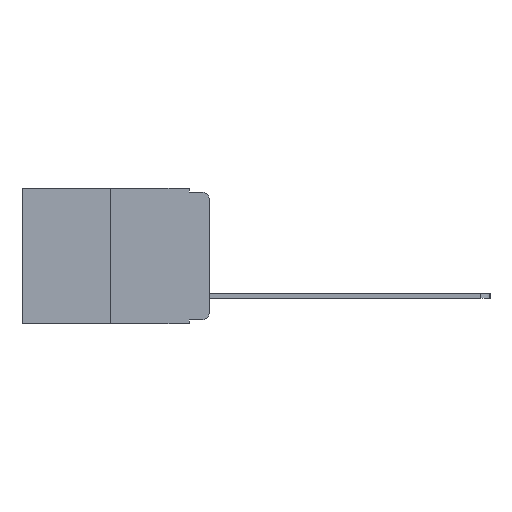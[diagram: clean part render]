
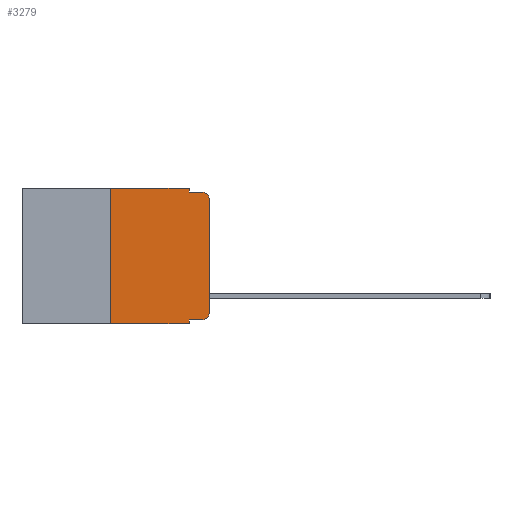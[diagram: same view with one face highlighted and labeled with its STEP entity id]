
A CAD part, left-side view. The second image highlights one B-rep face of the part: STEP entity #3279.
In plain terms, the highlighted planar face has unit normal (-1, 0, 0).
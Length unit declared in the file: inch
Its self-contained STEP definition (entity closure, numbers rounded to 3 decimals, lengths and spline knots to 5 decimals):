
#156 = CARTESIAN_POINT ( 'NONE',  ( 0., 0.02, -0.01 ) ) ;
#535 = ORIENTED_EDGE ( 'NONE', *, *, #969, .T. ) ;
#563 = CARTESIAN_POINT ( 'NONE',  ( 0., 0., -0.03 ) ) ;
#684 = VECTOR ( 'NONE', #9339, 39.37008 ) ;
#969 = EDGE_CURVE ( 'NONE', #7071, #10668, #7395, .T. ) ;
#1156 = VECTOR ( 'NONE', #9310, 39.37008 ) ;
#1168 = CARTESIAN_POINT ( 'NONE',  ( 0., 0.25, 0. ) ) ;
#1169 = VERTEX_POINT ( 'NONE', #3076 ) ;
#1619 = VERTEX_POINT ( 'NONE', #1168 ) ;
#1638 = FACE_OUTER_BOUND ( 'NONE', #4559, .T. ) ;
#1815 = CIRCLE ( 'NONE', #15956, 0.02 ) ;
#1949 = CARTESIAN_POINT ( 'NONE',  ( 0., 0.051, 0. ) ) ;
#2222 = ORIENTED_EDGE ( 'NONE', *, *, #12301, .F. ) ;
#2298 = LINE ( 'NONE', #12365, #6300 ) ;
#2747 = CARTESIAN_POINT ( 'NONE',  ( 0., 0., -0.313 ) ) ;
#2763 = DIRECTION ( 'NONE',  ( -1., 0., 0. ) ) ;
#2856 = LINE ( 'NONE', #8801, #13607 ) ;
#3076 = CARTESIAN_POINT ( 'NONE',  ( 0., 0.051, -0.333 ) ) ;
#3279 = ADVANCED_FACE ( 'NONE', ( #1638 ), #4726, .F. ) ;
#3405 = DIRECTION ( 'NONE',  ( 0., -1., 0. ) ) ;
#4073 = CARTESIAN_POINT ( 'NONE',  ( 0., 0.051, 0. ) ) ;
#4359 = EDGE_CURVE ( 'NONE', #1619, #12230, #13391, .T. ) ;
#4559 = EDGE_LOOP ( 'NONE', ( #16207, #16628, #2222, #13910, #7570, #8015, #535, #16010, #16838, #10166 ) ) ;
#4726 = PLANE ( 'NONE',  #13840 ) ;
#4734 = EDGE_CURVE ( 'NONE', #7071, #1619, #2856, .T. ) ;
#4788 = DIRECTION ( 'NONE',  ( 1., 0., 0. ) ) ;
#5229 = EDGE_CURVE ( 'NONE', #13430, #14707, #1815, .T. ) ;
#5599 = EDGE_CURVE ( 'NONE', #1169, #13430, #2298, .T. ) ;
#6300 = VECTOR ( 'NONE', #13684, 39.37008 ) ;
#6925 = EDGE_CURVE ( 'NONE', #1169, #10668, #13005, .T. ) ;
#7071 = VERTEX_POINT ( 'NONE', #15004 ) ;
#7157 = DIRECTION ( 'NONE',  ( 0., 0., -1. ) ) ;
#7208 = CARTESIAN_POINT ( 'NONE',  ( 0., 0.051, -0.01 ) ) ;
#7281 = LINE ( 'NONE', #12163, #10475 ) ;
#7308 = AXIS2_PLACEMENT_3D ( 'NONE', #16505, #8493, #7157 ) ;
#7395 = LINE ( 'NONE', #14921, #11018 ) ;
#7570 = ORIENTED_EDGE ( 'NONE', *, *, #4359, .F. ) ;
#7743 = CARTESIAN_POINT ( 'NONE',  ( 0., 0.02, -0.333 ) ) ;
#8015 = ORIENTED_EDGE ( 'NONE', *, *, #4734, .F. ) ;
#8082 = EDGE_CURVE ( 'NONE', #17076, #13344, #10045, .T. ) ;
#8493 = DIRECTION ( 'NONE',  ( -1., 0., 0. ) ) ;
#8608 = LINE ( 'NONE', #1949, #684 ) ;
#8801 = CARTESIAN_POINT ( 'NONE',  ( 0., 0.25, 0. ) ) ;
#9310 = DIRECTION ( 'NONE',  ( 0., 0., -1. ) ) ;
#9339 = DIRECTION ( 'NONE',  ( 0., 0., -1. ) ) ;
#10045 = CIRCLE ( 'NONE', #7308, 0.02 ) ;
#10166 = ORIENTED_EDGE ( 'NONE', *, *, #5229, .T. ) ;
#10178 = VERTEX_POINT ( 'NONE', #7208 ) ;
#10475 = VECTOR ( 'NONE', #13488, 39.37008 ) ;
#10668 = VERTEX_POINT ( 'NONE', #10711 ) ;
#10711 = CARTESIAN_POINT ( 'NONE',  ( 0., 0.051, -0.343 ) ) ;
#11018 = VECTOR ( 'NONE', #14616, 39.37008 ) ;
#11313 = CARTESIAN_POINT ( 'NONE',  ( 0., 0.02, -0.313 ) ) ;
#11963 = EDGE_CURVE ( 'NONE', #12230, #10178, #8608, .T. ) ;
#12059 = EDGE_CURVE ( 'NONE', #14707, #17076, #7281, .T. ) ;
#12163 = CARTESIAN_POINT ( 'NONE',  ( 0., 0., 0. ) ) ;
#12230 = VERTEX_POINT ( 'NONE', #4073 ) ;
#12301 = EDGE_CURVE ( 'NONE', #10178, #13344, #17746, .T. ) ;
#12365 = CARTESIAN_POINT ( 'NONE',  ( 0., 0.051, -0.333 ) ) ;
#12659 = DIRECTION ( 'NONE',  ( 0., 0., -1. ) ) ;
#12980 = VECTOR ( 'NONE', #3405, 39.37008 ) ;
#13005 = LINE ( 'NONE', #15967, #1156 ) ;
#13073 = CARTESIAN_POINT ( 'NONE',  ( 0., 0.473, 0. ) ) ;
#13344 = VERTEX_POINT ( 'NONE', #156 ) ;
#13391 = LINE ( 'NONE', #17128, #12980 ) ;
#13430 = VERTEX_POINT ( 'NONE', #7743 ) ;
#13488 = DIRECTION ( 'NONE',  ( 0., 0., 1. ) ) ;
#13607 = VECTOR ( 'NONE', #18087, 39.37008 ) ;
#13684 = DIRECTION ( 'NONE',  ( 0., -1., 0. ) ) ;
#13840 = AXIS2_PLACEMENT_3D ( 'NONE', #13073, #4788, #14390 ) ;
#13881 = DIRECTION ( 'NONE',  ( 0., -1., 0. ) ) ;
#13910 = ORIENTED_EDGE ( 'NONE', *, *, #11963, .F. ) ;
#14244 = VECTOR ( 'NONE', #13881, 39.37008 ) ;
#14390 = DIRECTION ( 'NONE',  ( 0., 0., -1. ) ) ;
#14616 = DIRECTION ( 'NONE',  ( 0., -1., 0. ) ) ;
#14707 = VERTEX_POINT ( 'NONE', #2747 ) ;
#14921 = CARTESIAN_POINT ( 'NONE',  ( 0., 0.473, -0.343 ) ) ;
#15004 = CARTESIAN_POINT ( 'NONE',  ( 0., 0.25, -0.343 ) ) ;
#15143 = CARTESIAN_POINT ( 'NONE',  ( 0., 0.051, -0.01 ) ) ;
#15956 = AXIS2_PLACEMENT_3D ( 'NONE', #11313, #2763, #12659 ) ;
#15967 = CARTESIAN_POINT ( 'NONE',  ( 0., 0.051, 0. ) ) ;
#16010 = ORIENTED_EDGE ( 'NONE', *, *, #6925, .F. ) ;
#16207 = ORIENTED_EDGE ( 'NONE', *, *, #12059, .T. ) ;
#16505 = CARTESIAN_POINT ( 'NONE',  ( 0., 0.02, -0.03 ) ) ;
#16628 = ORIENTED_EDGE ( 'NONE', *, *, #8082, .T. ) ;
#16838 = ORIENTED_EDGE ( 'NONE', *, *, #5599, .T. ) ;
#17076 = VERTEX_POINT ( 'NONE', #563 ) ;
#17128 = CARTESIAN_POINT ( 'NONE',  ( 0., 0.473, 0. ) ) ;
#17746 = LINE ( 'NONE', #15143, #14244 ) ;
#18087 = DIRECTION ( 'NONE',  ( 0., 0., 1. ) ) ;
